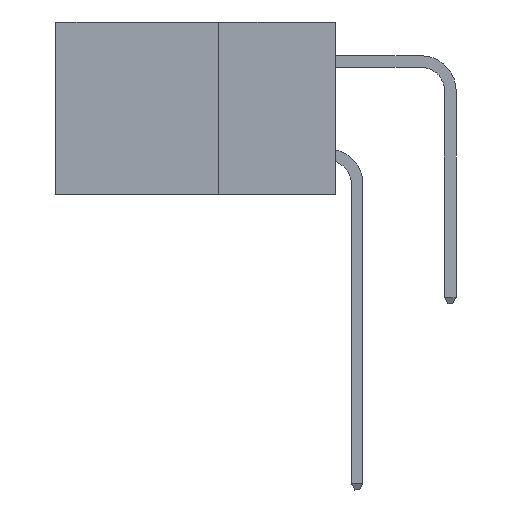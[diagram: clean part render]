
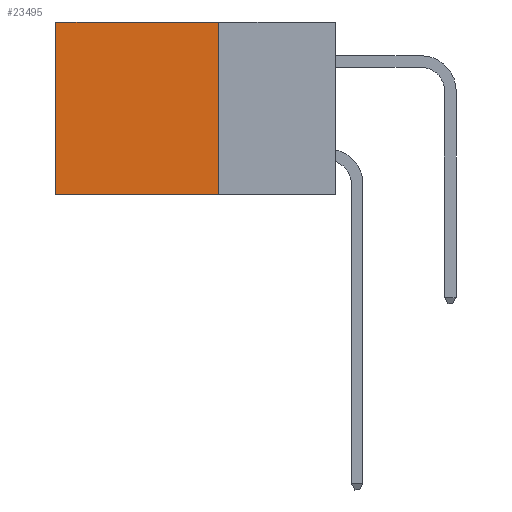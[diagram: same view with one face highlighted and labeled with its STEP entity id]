
A CAD part, left-side view. The second image highlights one B-rep face of the part: STEP entity #23495.
In plain terms, the highlighted planar face has unit normal (-1, 0, 0).
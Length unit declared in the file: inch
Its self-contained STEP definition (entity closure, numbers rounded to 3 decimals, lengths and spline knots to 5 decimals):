
#426 = DIRECTION ( 'NONE',  ( 0., 1., 0. ) ) ;
#2342 = LINE ( 'NONE', #38614, #38265 ) ;
#3834 = VECTOR ( 'NONE', #12253, 39.37008 ) ;
#5516 = CARTESIAN_POINT ( 'NONE',  ( 0.2875, 0.6, 0. ) ) ;
#12004 = DIRECTION ( 'NONE',  ( 0., 1., 0. ) ) ;
#12253 = DIRECTION ( 'NONE',  ( 0., 0., -1. ) ) ;
#13536 = EDGE_CURVE ( 'NONE', #23550, #28988, #16925, .T. ) ;
#14082 = ORIENTED_EDGE ( 'NONE', *, *, #32428, .F. ) ;
#15216 = VERTEX_POINT ( 'NONE', #42284 ) ;
#16925 = LINE ( 'NONE', #5516, #3834 ) ;
#17551 = VECTOR ( 'NONE', #40570, 39.37008 ) ;
#18246 = DIRECTION ( 'NONE',  ( 1., 0., 0. ) ) ;
#18634 = LINE ( 'NONE', #30263, #17551 ) ;
#18845 = CARTESIAN_POINT ( 'NONE',  ( 0.2875, 0.6, 0. ) ) ;
#19162 = CARTESIAN_POINT ( 'NONE',  ( 0.2875, 0.25, -0.37 ) ) ;
#21473 = FACE_OUTER_BOUND ( 'NONE', #25495, .T. ) ;
#22019 = ORIENTED_EDGE ( 'NONE', *, *, #37331, .F. ) ;
#22728 = VERTEX_POINT ( 'NONE', #28801 ) ;
#23495 = ADVANCED_FACE ( 'NONE', ( #21473 ), #24937, .F. ) ;
#23550 = VERTEX_POINT ( 'NONE', #18845 ) ;
#24937 = PLANE ( 'NONE',  #33206 ) ;
#25495 = EDGE_LOOP ( 'NONE', ( #35986, #22019, #14082, #25823 ) ) ;
#25823 = ORIENTED_EDGE ( 'NONE', *, *, #40297, .T. ) ;
#28578 = CARTESIAN_POINT ( 'NONE',  ( 0.2875, 0.25, 0. ) ) ;
#28801 = CARTESIAN_POINT ( 'NONE',  ( 0.2875, 0.25, -0.37 ) ) ;
#28988 = VERTEX_POINT ( 'NONE', #29141 ) ;
#29141 = CARTESIAN_POINT ( 'NONE',  ( 0.2875, 0.6, -0.37 ) ) ;
#30263 = CARTESIAN_POINT ( 'NONE',  ( 0.2875, 0.25, 0. ) ) ;
#32428 = EDGE_CURVE ( 'NONE', #15216, #22728, #18634, .T. ) ;
#33206 = AXIS2_PLACEMENT_3D ( 'NONE', #28578, #18246, #35704 ) ;
#35704 = DIRECTION ( 'NONE',  ( 0., 0., -1. ) ) ;
#35986 = ORIENTED_EDGE ( 'NONE', *, *, #13536, .T. ) ;
#37331 = EDGE_CURVE ( 'NONE', #22728, #28988, #44869, .T. ) ;
#38265 = VECTOR ( 'NONE', #426, 39.37008 ) ;
#38614 = CARTESIAN_POINT ( 'NONE',  ( 0.2875, 0.25, 0. ) ) ;
#40297 = EDGE_CURVE ( 'NONE', #15216, #23550, #2342, .T. ) ;
#40570 = DIRECTION ( 'NONE',  ( 0., 0., -1. ) ) ;
#42133 = VECTOR ( 'NONE', #12004, 39.37008 ) ;
#42284 = CARTESIAN_POINT ( 'NONE',  ( 0.2875, 0.25, 0. ) ) ;
#44869 = LINE ( 'NONE', #19162, #42133 ) ;
